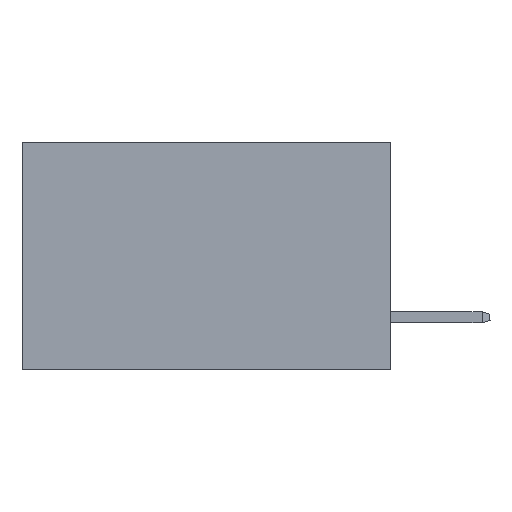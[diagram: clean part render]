
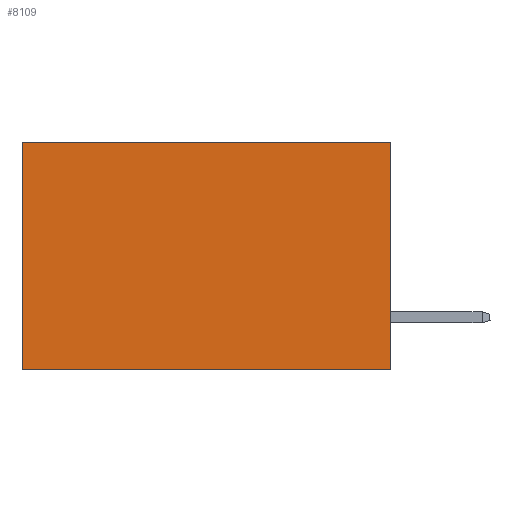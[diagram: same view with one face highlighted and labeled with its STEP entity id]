
A CAD part, left-side view. The second image highlights one B-rep face of the part: STEP entity #8109.
In plain terms, the highlighted planar face has unit normal (-1, 0, 0).
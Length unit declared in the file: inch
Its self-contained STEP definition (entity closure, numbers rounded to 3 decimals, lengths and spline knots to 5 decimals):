
#144 = EDGE_CURVE ( 'NONE', #39917, #11032, #3620, .T. ) ;
#1884 = DIRECTION ( 'NONE',  ( 0., 1., 0. ) ) ;
#3620 = LINE ( 'NONE', #9939, #39942 ) ;
#4916 = EDGE_CURVE ( 'NONE', #9101, #38528, #39745, .T. ) ;
#6952 = CARTESIAN_POINT ( 'NONE',  ( 0.2875, 0., 0. ) ) ;
#8109 = ADVANCED_FACE ( 'NONE', ( #24732 ), #16608, .F. ) ;
#9101 = VERTEX_POINT ( 'NONE', #6952 ) ;
#9939 = CARTESIAN_POINT ( 'NONE',  ( 0.2875, 0., -0.37 ) ) ;
#11032 = VERTEX_POINT ( 'NONE', #39493 ) ;
#11334 = LINE ( 'NONE', #33747, #32625 ) ;
#15395 = EDGE_CURVE ( 'NONE', #38528, #11032, #35466, .T. ) ;
#16219 = DIRECTION ( 'NONE',  ( 0., 0., -1. ) ) ;
#16608 = PLANE ( 'NONE',  #19391 ) ;
#17854 = DIRECTION ( 'NONE',  ( 0., 0., -1. ) ) ;
#18680 = DIRECTION ( 'NONE',  ( 0., 0., -1. ) ) ;
#18747 = ORIENTED_EDGE ( 'NONE', *, *, #144, .F. ) ;
#19391 = AXIS2_PLACEMENT_3D ( 'NONE', #35301, #34908, #16219 ) ;
#22893 = ORIENTED_EDGE ( 'NONE', *, *, #15395, .T. ) ;
#24215 = CARTESIAN_POINT ( 'NONE',  ( 0.2875, 0.6, 0. ) ) ;
#24732 = FACE_OUTER_BOUND ( 'NONE', #33937, .T. ) ;
#26255 = VECTOR ( 'NONE', #17854, 39.37008 ) ;
#27596 = CARTESIAN_POINT ( 'NONE',  ( 0.2875, 0., -0.37 ) ) ;
#28069 = DIRECTION ( 'NONE',  ( 0., 1., 0. ) ) ;
#31699 = EDGE_CURVE ( 'NONE', #9101, #39917, #11334, .T. ) ;
#32625 = VECTOR ( 'NONE', #18680, 39.37008 ) ;
#32840 = CARTESIAN_POINT ( 'NONE',  ( 0.2875, 0., 0. ) ) ;
#33747 = CARTESIAN_POINT ( 'NONE',  ( 0.2875, 0., 0. ) ) ;
#33937 = EDGE_LOOP ( 'NONE', ( #22893, #18747, #36262, #34857 ) ) ;
#34857 = ORIENTED_EDGE ( 'NONE', *, *, #4916, .T. ) ;
#34908 = DIRECTION ( 'NONE',  ( 1., 0., 0. ) ) ;
#35301 = CARTESIAN_POINT ( 'NONE',  ( 0.2875, 0., 0. ) ) ;
#35466 = LINE ( 'NONE', #24215, #26255 ) ;
#35861 = VECTOR ( 'NONE', #1884, 39.37008 ) ;
#36262 = ORIENTED_EDGE ( 'NONE', *, *, #31699, .F. ) ;
#38528 = VERTEX_POINT ( 'NONE', #38865 ) ;
#38865 = CARTESIAN_POINT ( 'NONE',  ( 0.2875, 0.6, 0. ) ) ;
#39493 = CARTESIAN_POINT ( 'NONE',  ( 0.2875, 0.6, -0.37 ) ) ;
#39745 = LINE ( 'NONE', #32840, #35861 ) ;
#39917 = VERTEX_POINT ( 'NONE', #27596 ) ;
#39942 = VECTOR ( 'NONE', #28069, 39.37008 ) ;
